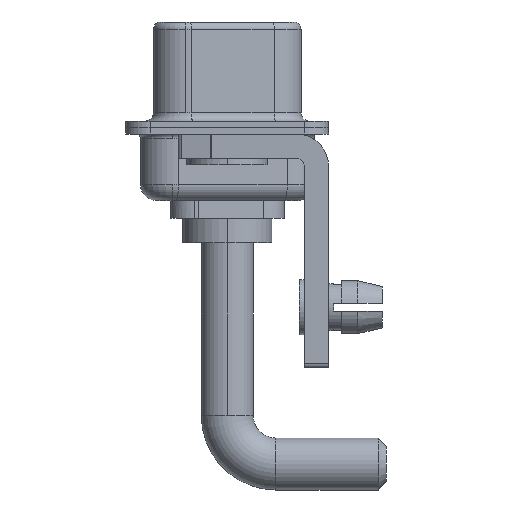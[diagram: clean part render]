
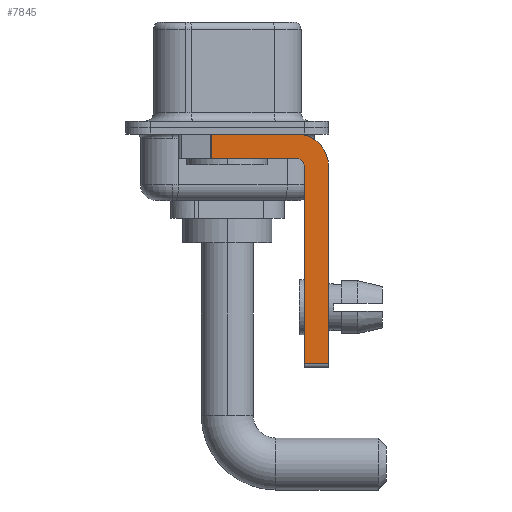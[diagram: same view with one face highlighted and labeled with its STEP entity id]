
A CAD part, left-side view. The second image highlights one B-rep face of the part: STEP entity #7845.
In plain terms, the highlighted planar face has unit normal (-1, 0, 0).
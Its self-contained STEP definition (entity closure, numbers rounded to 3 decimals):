
#23 = CARTESIAN_POINT ( 'NONE',  ( -2.9, -6.25, -2.4 ) ) ;
#25 = VERTEX_POINT ( 'NONE', #3436 ) ;
#270 = LINE ( 'NONE', #23, #5019 ) ;
#288 = CARTESIAN_POINT ( 'NONE',  ( -2.9, 3., -0.4 ) ) ;
#671 = EDGE_CURVE ( 'NONE', #6368, #14150, #15007, .T. ) ;
#688 = VERTEX_POINT ( 'NONE', #5830 ) ;
#834 = CARTESIAN_POINT ( 'NONE',  ( -2.9, 0.978, -0.4 ) ) ;
#1426 = AXIS2_PLACEMENT_3D ( 'NONE', #14390, #1480, #6655 ) ;
#1447 = EDGE_CURVE ( 'NONE', #25, #688, #270, .T. ) ;
#1480 = DIRECTION ( 'NONE',  ( 1., 0., 0. ) ) ;
#1622 = ORIENTED_EDGE ( 'NONE', *, *, #1447, .F. ) ;
#1953 = DIRECTION ( 'NONE',  ( 0., -1., 0. ) ) ;
#2597 = VERTEX_POINT ( 'NONE', #3127 ) ;
#2679 = ORIENTED_EDGE ( 'NONE', *, *, #671, .F. ) ;
#2960 = EDGE_CURVE ( 'NONE', #11205, #10264, #3015, .T. ) ;
#3009 = DIRECTION ( 'NONE',  ( 0., 0., -1. ) ) ;
#3015 = LINE ( 'NONE', #288, #6480 ) ;
#3127 = CARTESIAN_POINT ( 'NONE',  ( -2.9, -4.75, -14.55 ) ) ;
#3436 = CARTESIAN_POINT ( 'NONE',  ( -2.9, -6.25, -2.4 ) ) ;
#4127 = DIRECTION ( 'NONE',  ( -1., 0., 0. ) ) ;
#4290 = ORIENTED_EDGE ( 'NONE', *, *, #7825, .F. ) ;
#4382 = DIRECTION ( 'NONE',  ( 0., 0., 1. ) ) ;
#4497 = VECTOR ( 'NONE', #6791, 1000. ) ;
#4538 = ORIENTED_EDGE ( 'NONE', *, *, #11108, .F. ) ;
#4552 = VECTOR ( 'NONE', #12612, 1000. ) ;
#4858 = CARTESIAN_POINT ( 'NONE',  ( -2.9, 0.978, -1.9 ) ) ;
#5019 = VECTOR ( 'NONE', #10564, 1000. ) ;
#5830 = CARTESIAN_POINT ( 'NONE',  ( -2.9, -6.25, -14.55 ) ) ;
#6368 = VERTEX_POINT ( 'NONE', #10562 ) ;
#6480 = VECTOR ( 'NONE', #16396, 1000. ) ;
#6655 = DIRECTION ( 'NONE',  ( 0., 0., -1. ) ) ;
#6791 = DIRECTION ( 'NONE',  ( 0., 0., 1. ) ) ;
#7135 = AXIS2_PLACEMENT_3D ( 'NONE', #12111, #11853, #3009 ) ;
#7311 = EDGE_CURVE ( 'NONE', #11783, #6368, #15822, .T. ) ;
#7591 = ORIENTED_EDGE ( 'NONE', *, *, #2960, .F. ) ;
#7825 = EDGE_CURVE ( 'NONE', #10264, #25, #8225, .T. ) ;
#7845 = ADVANCED_FACE ( 'NONE', ( #10491 ), #9226, .F. ) ;
#8225 = CIRCLE ( 'NONE', #7135, 2. ) ;
#8490 = DIRECTION ( 'NONE',  ( 0., 1., 0. ) ) ;
#8839 = VECTOR ( 'NONE', #8490, 1000. ) ;
#9226 = PLANE ( 'NONE',  #1426 ) ;
#9518 = CARTESIAN_POINT ( 'NONE',  ( -2.9, -4.25, -1.9 ) ) ;
#9738 = ORIENTED_EDGE ( 'NONE', *, *, #7311, .F. ) ;
#10264 = VERTEX_POINT ( 'NONE', #10685 ) ;
#10491 = FACE_OUTER_BOUND ( 'NONE', #14394, .T. ) ;
#10562 = CARTESIAN_POINT ( 'NONE',  ( -2.9, -4.25, -1.9 ) ) ;
#10564 = DIRECTION ( 'NONE',  ( 0., 0., -1. ) ) ;
#10685 = CARTESIAN_POINT ( 'NONE',  ( -2.9, -4.25, -0.4 ) ) ;
#10934 = CARTESIAN_POINT ( 'NONE',  ( -2.9, -4.25, -2.4 ) ) ;
#11108 = EDGE_CURVE ( 'NONE', #2597, #11783, #14352, .T. ) ;
#11205 = VERTEX_POINT ( 'NONE', #834 ) ;
#11426 = ORIENTED_EDGE ( 'NONE', *, *, #15220, .T. ) ;
#11783 = VERTEX_POINT ( 'NONE', #14917 ) ;
#11853 = DIRECTION ( 'NONE',  ( 1., 0., 0. ) ) ;
#12051 = ORIENTED_EDGE ( 'NONE', *, *, #14470, .T. ) ;
#12111 = CARTESIAN_POINT ( 'NONE',  ( -2.9, -4.25, -2.4 ) ) ;
#12359 = CARTESIAN_POINT ( 'NONE',  ( -2.9, 0.978, -1.9 ) ) ;
#12531 = LINE ( 'NONE', #12359, #4552 ) ;
#12612 = DIRECTION ( 'NONE',  ( 0., 0., -1. ) ) ;
#13683 = CARTESIAN_POINT ( 'NONE',  ( -2.9, -4.25, -14.55 ) ) ;
#14150 = VERTEX_POINT ( 'NONE', #4858 ) ;
#14352 = LINE ( 'NONE', #14688, #4497 ) ;
#14390 = CARTESIAN_POINT ( 'NONE',  ( -2.9, -4.25, -2.4 ) ) ;
#14394 = EDGE_LOOP ( 'NONE', ( #7591, #11426, #2679, #9738, #4538, #12051, #1622, #4290 ) ) ;
#14470 = EDGE_CURVE ( 'NONE', #2597, #688, #16044, .T. ) ;
#14563 = VECTOR ( 'NONE', #1953, 1000. ) ;
#14688 = CARTESIAN_POINT ( 'NONE',  ( -2.9, -4.75, -14.8 ) ) ;
#14917 = CARTESIAN_POINT ( 'NONE',  ( -2.9, -4.75, -2.4 ) ) ;
#15007 = LINE ( 'NONE', #9518, #8839 ) ;
#15024 = AXIS2_PLACEMENT_3D ( 'NONE', #10934, #4127, #4382 ) ;
#15220 = EDGE_CURVE ( 'NONE', #11205, #14150, #12531, .T. ) ;
#15822 = CIRCLE ( 'NONE', #15024, 0.5 ) ;
#16044 = LINE ( 'NONE', #13683, #14563 ) ;
#16396 = DIRECTION ( 'NONE',  ( 0., -1., 0. ) ) ;
